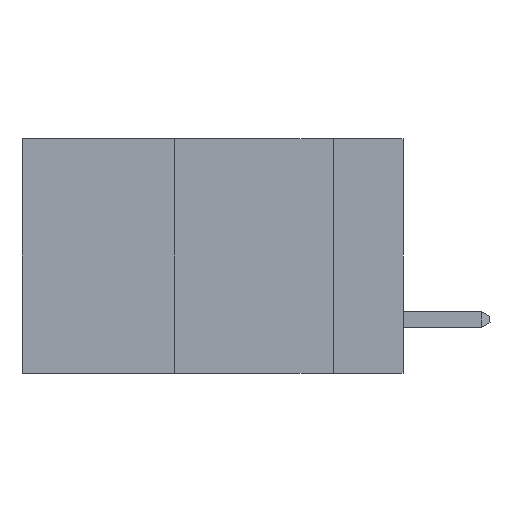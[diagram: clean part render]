
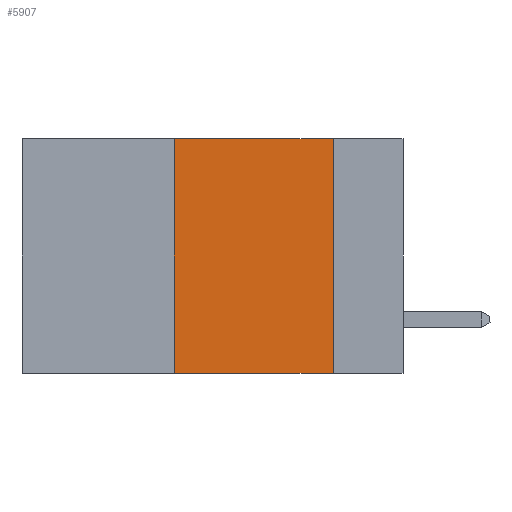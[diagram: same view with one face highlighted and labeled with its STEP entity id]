
A CAD part, left-side view. The second image highlights one B-rep face of the part: STEP entity #5907.
In plain terms, the highlighted planar face has unit normal (-1, 0, 0).
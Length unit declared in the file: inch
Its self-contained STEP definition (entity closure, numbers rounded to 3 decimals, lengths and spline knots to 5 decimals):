
#33 = LINE ( 'NONE', #4903, #4274 ) ;
#420 = VERTEX_POINT ( 'NONE', #9048 ) ;
#668 = VECTOR ( 'NONE', #7995, 39.37008 ) ;
#868 = EDGE_CURVE ( 'NONE', #4438, #420, #5506, .T. ) ;
#994 = ORIENTED_EDGE ( 'NONE', *, *, #3624, .F. ) ;
#2006 = EDGE_CURVE ( 'NONE', #8856, #5179, #7761, .T. ) ;
#2192 = CARTESIAN_POINT ( 'NONE',  ( 0., 0.11, 0. ) ) ;
#2909 = ORIENTED_EDGE ( 'NONE', *, *, #868, .T. ) ;
#3172 = VECTOR ( 'NONE', #7156, 39.37008 ) ;
#3212 = LINE ( 'NONE', #2192, #668 ) ;
#3498 = DIRECTION ( 'NONE',  ( 0., -1., 0. ) ) ;
#3574 = AXIS2_PLACEMENT_3D ( 'NONE', #8714, #9487, #7244 ) ;
#3624 = EDGE_CURVE ( 'NONE', #4438, #8856, #33, .T. ) ;
#4274 = VECTOR ( 'NONE', #4886, 39.37008 ) ;
#4434 = CARTESIAN_POINT ( 'NONE',  ( 0., 0.6, 0. ) ) ;
#4438 = VERTEX_POINT ( 'NONE', #8361 ) ;
#4886 = DIRECTION ( 'NONE',  ( 0., 0., 1. ) ) ;
#4903 = CARTESIAN_POINT ( 'NONE',  ( 0., 0.36, 0. ) ) ;
#5026 = PLANE ( 'NONE',  #3574 ) ;
#5179 = VERTEX_POINT ( 'NONE', #8916 ) ;
#5325 = ORIENTED_EDGE ( 'NONE', *, *, #7437, .F. ) ;
#5506 = LINE ( 'NONE', #6858, #3172 ) ;
#5855 = EDGE_LOOP ( 'NONE', ( #5325, #6014, #994, #2909 ) ) ;
#5907 = ADVANCED_FACE ( 'NONE', ( #6763 ), #5026, .F. ) ;
#6014 = ORIENTED_EDGE ( 'NONE', *, *, #2006, .F. ) ;
#6763 = FACE_OUTER_BOUND ( 'NONE', #5855, .T. ) ;
#6858 = CARTESIAN_POINT ( 'NONE',  ( 0., 0.6, -0.37 ) ) ;
#7156 = DIRECTION ( 'NONE',  ( 0., -1., 0. ) ) ;
#7244 = DIRECTION ( 'NONE',  ( 0., 0., -1. ) ) ;
#7437 = EDGE_CURVE ( 'NONE', #5179, #420, #3212, .T. ) ;
#7761 = LINE ( 'NONE', #4434, #9182 ) ;
#7995 = DIRECTION ( 'NONE',  ( 0., 0., -1. ) ) ;
#8361 = CARTESIAN_POINT ( 'NONE',  ( 0., 0.36, -0.37 ) ) ;
#8620 = CARTESIAN_POINT ( 'NONE',  ( 0., 0.36, 0. ) ) ;
#8714 = CARTESIAN_POINT ( 'NONE',  ( 0., 0.6, 0. ) ) ;
#8856 = VERTEX_POINT ( 'NONE', #8620 ) ;
#8916 = CARTESIAN_POINT ( 'NONE',  ( 0., 0.11, 0. ) ) ;
#9048 = CARTESIAN_POINT ( 'NONE',  ( 0., 0.11, -0.37 ) ) ;
#9182 = VECTOR ( 'NONE', #3498, 39.37008 ) ;
#9487 = DIRECTION ( 'NONE',  ( 1., 0., 0. ) ) ;
